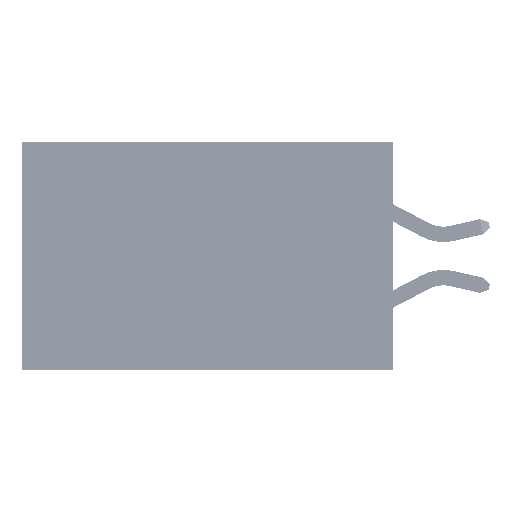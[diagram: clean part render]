
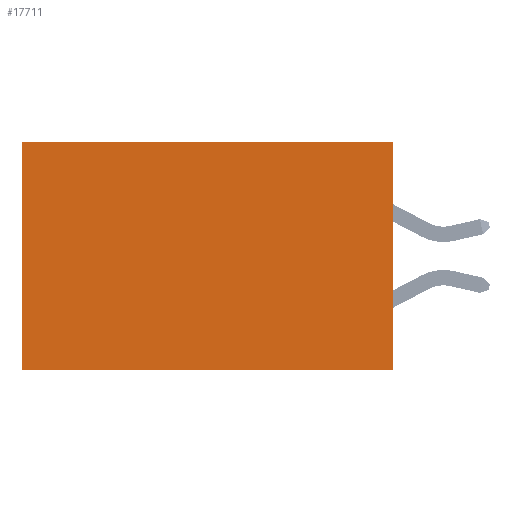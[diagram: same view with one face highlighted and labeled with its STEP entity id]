
A CAD part, left-side view. The second image highlights one B-rep face of the part: STEP entity #17711.
In plain terms, the highlighted planar face has unit normal (-1, 0, 0).
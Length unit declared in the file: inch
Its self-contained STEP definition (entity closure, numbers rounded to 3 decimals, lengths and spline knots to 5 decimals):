
#787 = DIRECTION ( 'NONE',  ( 0., 1., 0. ) ) ;
#1561 = LINE ( 'NONE', #8131, #20504 ) ;
#1617 = DIRECTION ( 'NONE',  ( 0., 0., -1. ) ) ;
#1812 = LINE ( 'NONE', #49262, #49874 ) ;
#2358 = VERTEX_POINT ( 'NONE', #42554 ) ;
#2513 = EDGE_LOOP ( 'NONE', ( #34673, #41158, #22474, #10917 ) ) ;
#6836 = DIRECTION ( 'NONE',  ( 0., 0., -1. ) ) ;
#8131 = CARTESIAN_POINT ( 'NONE',  ( 0.2875, 0., 0. ) ) ;
#10917 = ORIENTED_EDGE ( 'NONE', *, *, #27565, .T. ) ;
#12207 = DIRECTION ( 'NONE',  ( 0., 1., 0. ) ) ;
#15803 = VERTEX_POINT ( 'NONE', #33918 ) ;
#16862 = AXIS2_PLACEMENT_3D ( 'NONE', #26280, #33923, #30205 ) ;
#17711 = ADVANCED_FACE ( 'NONE', ( #22425 ), #42227, .F. ) ;
#18300 = CARTESIAN_POINT ( 'NONE',  ( 0.2875, 0.6, 0. ) ) ;
#18332 = EDGE_CURVE ( 'NONE', #15803, #46255, #1812, .T. ) ;
#20504 = VECTOR ( 'NONE', #12207, 39.37008 ) ;
#22425 = FACE_OUTER_BOUND ( 'NONE', #2513, .T. ) ;
#22474 = ORIENTED_EDGE ( 'NONE', *, *, #39242, .F. ) ;
#23557 = VECTOR ( 'NONE', #1617, 39.37008 ) ;
#23918 = LINE ( 'NONE', #31260, #49937 ) ;
#24628 = VERTEX_POINT ( 'NONE', #18300 ) ;
#26280 = CARTESIAN_POINT ( 'NONE',  ( 0.2875, 0., 0. ) ) ;
#27565 = EDGE_CURVE ( 'NONE', #2358, #24628, #1561, .T. ) ;
#28368 = CARTESIAN_POINT ( 'NONE',  ( 0.2875, 0.6, -0.37 ) ) ;
#30205 = DIRECTION ( 'NONE',  ( 0., 0., -1. ) ) ;
#31260 = CARTESIAN_POINT ( 'NONE',  ( 0.2875, 0.6, 0. ) ) ;
#33918 = CARTESIAN_POINT ( 'NONE',  ( 0.2875, 0., -0.37 ) ) ;
#33923 = DIRECTION ( 'NONE',  ( 1., 0., 0. ) ) ;
#34356 = CARTESIAN_POINT ( 'NONE',  ( 0.2875, 0., 0. ) ) ;
#34673 = ORIENTED_EDGE ( 'NONE', *, *, #47397, .T. ) ;
#38803 = LINE ( 'NONE', #34356, #23557 ) ;
#39242 = EDGE_CURVE ( 'NONE', #2358, #15803, #38803, .T. ) ;
#41158 = ORIENTED_EDGE ( 'NONE', *, *, #18332, .F. ) ;
#42227 = PLANE ( 'NONE',  #16862 ) ;
#42554 = CARTESIAN_POINT ( 'NONE',  ( 0.2875, 0., 0. ) ) ;
#46255 = VERTEX_POINT ( 'NONE', #28368 ) ;
#47397 = EDGE_CURVE ( 'NONE', #24628, #46255, #23918, .T. ) ;
#49262 = CARTESIAN_POINT ( 'NONE',  ( 0.2875, 0., -0.37 ) ) ;
#49874 = VECTOR ( 'NONE', #787, 39.37008 ) ;
#49937 = VECTOR ( 'NONE', #6836, 39.37008 ) ;
